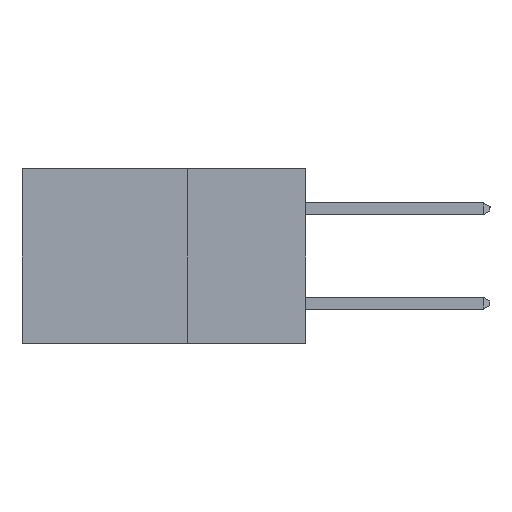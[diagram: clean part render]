
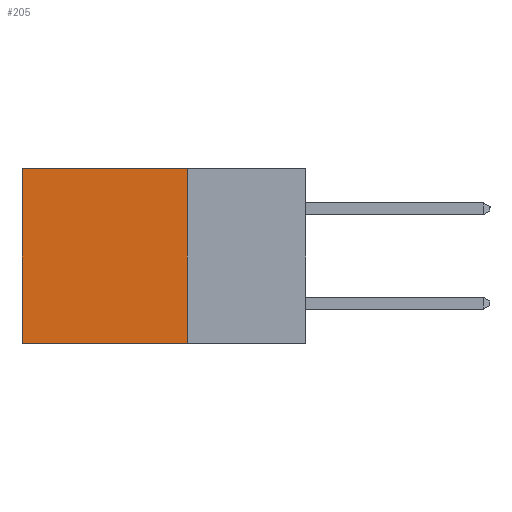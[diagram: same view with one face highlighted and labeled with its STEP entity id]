
A CAD part, left-side view. The second image highlights one B-rep face of the part: STEP entity #205.
In plain terms, the highlighted planar face has unit normal (-1, 0, 0).
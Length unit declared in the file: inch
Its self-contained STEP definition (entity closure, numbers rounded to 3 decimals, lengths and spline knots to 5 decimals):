
#205 = ADVANCED_FACE ( 'NONE', ( #13218 ), #15803, .F. ) ;
#381 = LINE ( 'NONE', #5510, #1703 ) ;
#703 = ORIENTED_EDGE ( 'NONE', *, *, #16028, .T. ) ;
#1389 = VECTOR ( 'NONE', #6185, 39.37008 ) ;
#1703 = VECTOR ( 'NONE', #16105, 39.37008 ) ;
#2083 = ORIENTED_EDGE ( 'NONE', *, *, #13418, .F. ) ;
#2345 = VERTEX_POINT ( 'NONE', #4809 ) ;
#3532 = LINE ( 'NONE', #4553, #1389 ) ;
#4553 = CARTESIAN_POINT ( 'NONE',  ( 0.2615, 0.25, -0.37 ) ) ;
#4809 = CARTESIAN_POINT ( 'NONE',  ( 0.2615, 0.6, -0.37 ) ) ;
#4870 = LINE ( 'NONE', #10056, #15712 ) ;
#5302 = DIRECTION ( 'NONE',  ( 1., 0., 0. ) ) ;
#5330 = DIRECTION ( 'NONE',  ( 0., 0., -1. ) ) ;
#5463 = DIRECTION ( 'NONE',  ( 0., 0., -1. ) ) ;
#5510 = CARTESIAN_POINT ( 'NONE',  ( 0.2615, 0.25, 0. ) ) ;
#6185 = DIRECTION ( 'NONE',  ( 0., 1., 0. ) ) ;
#6213 = CARTESIAN_POINT ( 'NONE',  ( 0.2615, 0.25, 0. ) ) ;
#6461 = CARTESIAN_POINT ( 'NONE',  ( 0.2615, 0.25, -0.37 ) ) ;
#6463 = VECTOR ( 'NONE', #5330, 39.37008 ) ;
#6465 = CARTESIAN_POINT ( 'NONE',  ( 0.2615, 0.25, -0.37 ) ) ;
#6718 = LINE ( 'NONE', #6465, #6463 ) ;
#7673 = AXIS2_PLACEMENT_3D ( 'NONE', #13064, #5302, #5463 ) ;
#9774 = EDGE_LOOP ( 'NONE', ( #12884, #2083, #16608, #703 ) ) ;
#10056 = CARTESIAN_POINT ( 'NONE',  ( 0.2615, 0.6, -0.37 ) ) ;
#10705 = EDGE_CURVE ( 'NONE', #16112, #16302, #6718, .T. ) ;
#11095 = EDGE_CURVE ( 'NONE', #13482, #2345, #4870, .T. ) ;
#12884 = ORIENTED_EDGE ( 'NONE', *, *, #11095, .T. ) ;
#13064 = CARTESIAN_POINT ( 'NONE',  ( 0.2615, 0.25, -0.37 ) ) ;
#13218 = FACE_OUTER_BOUND ( 'NONE', #9774, .T. ) ;
#13418 = EDGE_CURVE ( 'NONE', #16302, #2345, #3532, .T. ) ;
#13482 = VERTEX_POINT ( 'NONE', #16548 ) ;
#15267 = DIRECTION ( 'NONE',  ( 0., 0., -1. ) ) ;
#15712 = VECTOR ( 'NONE', #15267, 39.37008 ) ;
#15803 = PLANE ( 'NONE',  #7673 ) ;
#16028 = EDGE_CURVE ( 'NONE', #16112, #13482, #381, .T. ) ;
#16105 = DIRECTION ( 'NONE',  ( 0., 1., 0. ) ) ;
#16112 = VERTEX_POINT ( 'NONE', #6213 ) ;
#16302 = VERTEX_POINT ( 'NONE', #6461 ) ;
#16548 = CARTESIAN_POINT ( 'NONE',  ( 0.2615, 0.6, 0. ) ) ;
#16608 = ORIENTED_EDGE ( 'NONE', *, *, #10705, .F. ) ;
